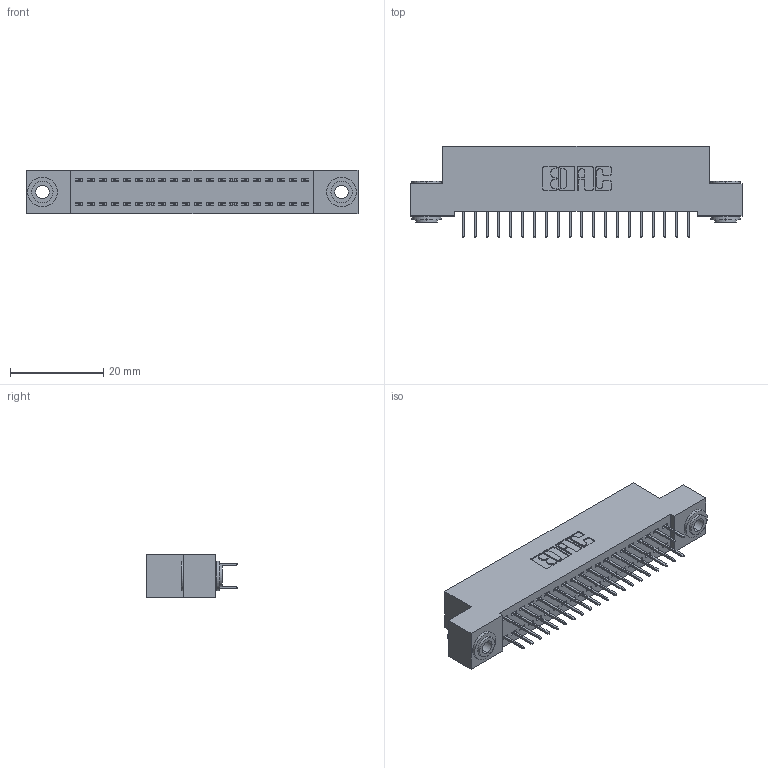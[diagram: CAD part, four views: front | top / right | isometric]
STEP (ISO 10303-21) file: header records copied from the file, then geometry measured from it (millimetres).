
FILE_DESCRIPTION (( 'STEP AP203' ), '1' );
FILE_NAME ('392-040-524-203.STEP', '2019-10-07T19:53:07', ( '' ), ( '' ), 'SwSTEP 2.0', 'SolidWorks 2016', '' );
FILE_SCHEMA (( 'CONFIG_CONTROL_DESIGN' ));
Length unit declared in the file: inch
Products named in the file (4): 345-292-001_345-293-124; 342-250-002_345-250-002-102; 392-040-524-203; 342 Part_.156 TH
Assembly tree (43 placements, depth 2):
  392-040-524-203
    342 Part_.156 TH
    345-292-001_345-293-124  x40
    342-250-002_345-250-002-102  x2
Bounding box: 71.12 x 19.69 x 9.4 mm (x, y, z)
Volume: 6248.3 mm3; surface area: 9685.2 mm2
Topology: 43 solids, 43 shells, 2388 faces, 6735 edges, 4326 vertices
Faces by surface type: plane 1756, cylinder 624, cone 8
Entity records: 16304 total; most frequent: CARTESIAN_POINT 2701, ORIENTED_EDGE 2630, DIRECTION 2381, EDGE_CURVE 1315, VECTOR 1167, LINE 1167, VERTEX_POINT 870, AXIS2_PLACEMENT_3D 607
